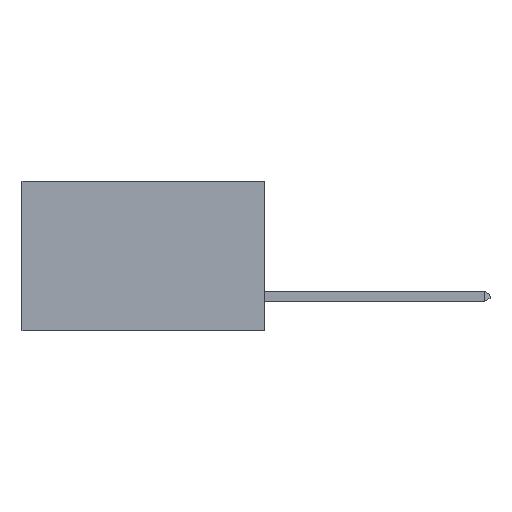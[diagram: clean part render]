
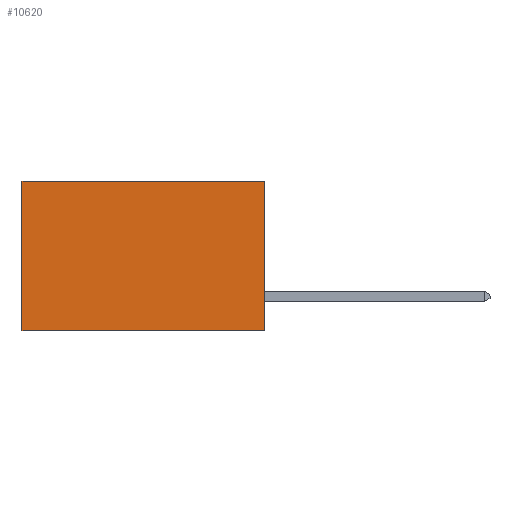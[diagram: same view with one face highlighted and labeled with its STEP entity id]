
A CAD part, left-side view. The second image highlights one B-rep face of the part: STEP entity #10620.
In plain terms, the highlighted planar face has unit normal (-1, 0, 0).
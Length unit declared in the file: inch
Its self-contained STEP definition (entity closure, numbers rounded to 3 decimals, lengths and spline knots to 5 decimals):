
#160 = FACE_OUTER_BOUND ( 'NONE', #24664, .T. ) ;
#182 = VECTOR ( 'NONE', #1379, 39.37008 ) ;
#434 = VECTOR ( 'NONE', #11581, 39.37008 ) ;
#1379 = DIRECTION ( 'NONE',  ( 0., 1., 0. ) ) ;
#1523 = LINE ( 'NONE', #24843, #6664 ) ;
#2949 = VERTEX_POINT ( 'NONE', #11307 ) ;
#4138 = VECTOR ( 'NONE', #14606, 39.37008 ) ;
#4760 = EDGE_CURVE ( 'NONE', #13498, #9393, #1523, .T. ) ;
#5866 = PLANE ( 'NONE',  #9883 ) ;
#6664 = VECTOR ( 'NONE', #25305, 39.37008 ) ;
#8058 = CARTESIAN_POINT ( 'NONE',  ( 0.298, 0., 0. ) ) ;
#8505 = CARTESIAN_POINT ( 'NONE',  ( 0.298, 0.6, 0. ) ) ;
#9393 = VERTEX_POINT ( 'NONE', #24571 ) ;
#9527 = EDGE_CURVE ( 'NONE', #9393, #2949, #18171, .T. ) ;
#9883 = AXIS2_PLACEMENT_3D ( 'NONE', #8058, #10232, #25175 ) ;
#10232 = DIRECTION ( 'NONE',  ( 1., 0., 0. ) ) ;
#10620 = ADVANCED_FACE ( 'NONE', ( #160 ), #5866, .F. ) ;
#11307 = CARTESIAN_POINT ( 'NONE',  ( 0.298, 0.6, -0.37 ) ) ;
#11368 = LINE ( 'NONE', #24379, #434 ) ;
#11427 = ORIENTED_EDGE ( 'NONE', *, *, #4760, .F. ) ;
#11581 = DIRECTION ( 'NONE',  ( 0., 1., 0. ) ) ;
#12460 = CARTESIAN_POINT ( 'NONE',  ( 0.298, 0.6, 0. ) ) ;
#12520 = ORIENTED_EDGE ( 'NONE', *, *, #15213, .T. ) ;
#13498 = VERTEX_POINT ( 'NONE', #14102 ) ;
#14102 = CARTESIAN_POINT ( 'NONE',  ( 0.298, 0., 0. ) ) ;
#14606 = DIRECTION ( 'NONE',  ( 0., 0., -1. ) ) ;
#15213 = EDGE_CURVE ( 'NONE', #13498, #19785, #11368, .T. ) ;
#15689 = ORIENTED_EDGE ( 'NONE', *, *, #22912, .T. ) ;
#18171 = LINE ( 'NONE', #22898, #182 ) ;
#19785 = VERTEX_POINT ( 'NONE', #8505 ) ;
#21273 = LINE ( 'NONE', #12460, #4138 ) ;
#22898 = CARTESIAN_POINT ( 'NONE',  ( 0.298, 0., -0.37 ) ) ;
#22912 = EDGE_CURVE ( 'NONE', #19785, #2949, #21273, .T. ) ;
#24379 = CARTESIAN_POINT ( 'NONE',  ( 0.298, 0., 0. ) ) ;
#24571 = CARTESIAN_POINT ( 'NONE',  ( 0.298, 0., -0.37 ) ) ;
#24664 = EDGE_LOOP ( 'NONE', ( #15689, #25822, #11427, #12520 ) ) ;
#24843 = CARTESIAN_POINT ( 'NONE',  ( 0.298, 0., 0. ) ) ;
#25175 = DIRECTION ( 'NONE',  ( 0., 0., -1. ) ) ;
#25305 = DIRECTION ( 'NONE',  ( 0., 0., -1. ) ) ;
#25822 = ORIENTED_EDGE ( 'NONE', *, *, #9527, .F. ) ;
